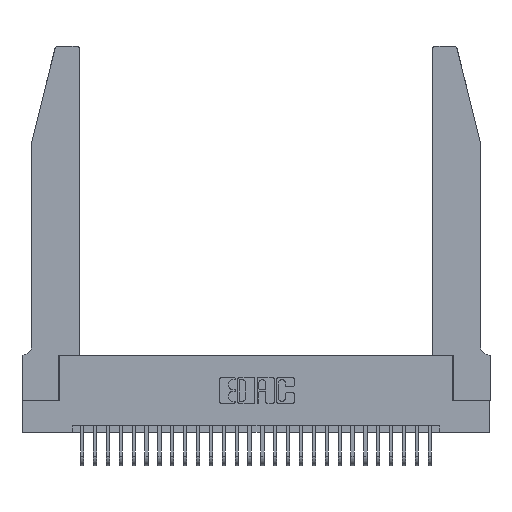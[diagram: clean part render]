
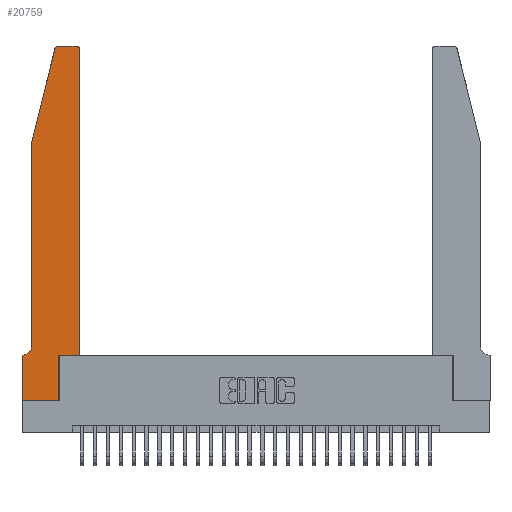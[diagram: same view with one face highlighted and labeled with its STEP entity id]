
A CAD part, top view. The second image highlights one B-rep face of the part: STEP entity #20759.
In plain terms, the highlighted planar face has unit normal (0, 0, 1).
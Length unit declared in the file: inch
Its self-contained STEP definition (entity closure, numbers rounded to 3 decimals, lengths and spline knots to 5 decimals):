
#238 = DIRECTION ( 'NONE',  ( 0., -1., 0. ) ) ;
#245 = CARTESIAN_POINT ( 'NONE',  ( 0.284, 2.72, 0.37 ) ) ;
#687 = VECTOR ( 'NONE', #22631, 39.37008 ) ;
#832 = CARTESIAN_POINT ( 'NONE',  ( 0.2865, 0.35, 0.37 ) ) ;
#835 = VERTEX_POINT ( 'NONE', #6418 ) ;
#898 = AXIS2_PLACEMENT_3D ( 'NONE', #245, #15365, #2438 ) ;
#1307 = VECTOR ( 'NONE', #238, 39.37008 ) ;
#1359 = LINE ( 'NONE', #5441, #687 ) ;
#1474 = EDGE_CURVE ( 'NONE', #16273, #2423, #24915, .T. ) ;
#1587 = ORIENTED_EDGE ( 'NONE', *, *, #12725, .T. ) ;
#1673 = EDGE_CURVE ( 'NONE', #17619, #4056, #3754, .T. ) ;
#2088 = VECTOR ( 'NONE', #20787, 39.37008 ) ;
#2423 = VERTEX_POINT ( 'NONE', #12526 ) ;
#2438 = DIRECTION ( 'NONE',  ( 1., 0., 0. ) ) ;
#2525 = ORIENTED_EDGE ( 'NONE', *, *, #5178, .T. ) ;
#2668 = DIRECTION ( 'NONE',  ( 0., 1., 0. ) ) ;
#2673 = DIRECTION ( 'NONE',  ( 1., 0., 0. ) ) ;
#2699 = VERTEX_POINT ( 'NONE', #11519 ) ;
#2999 = EDGE_LOOP ( 'NONE', ( #14582, #3633, #5471, #1587, #21951, #20219, #9209, #8102, #14599, #9055, #26476, #2525 ) ) ;
#3405 = VECTOR ( 'NONE', #24109, 39.37008 ) ;
#3633 = ORIENTED_EDGE ( 'NONE', *, *, #8452, .T. ) ;
#3653 = CIRCLE ( 'NONE', #20707, 0.03 ) ;
#3754 = LINE ( 'NONE', #13445, #5108 ) ;
#3864 = CIRCLE ( 'NONE', #7303, 0.07 ) ;
#3934 = EDGE_CURVE ( 'NONE', #6554, #13724, #21554, .T. ) ;
#4013 = VERTEX_POINT ( 'NONE', #22145 ) ;
#4056 = VERTEX_POINT ( 'NONE', #9401 ) ;
#4520 = CARTESIAN_POINT ( 'NONE',  ( 0.4205, 2.72, 0.37 ) ) ;
#4682 = VERTEX_POINT ( 'NONE', #832 ) ;
#5108 = VECTOR ( 'NONE', #2668, 39.37008 ) ;
#5178 = EDGE_CURVE ( 'NONE', #4056, #835, #3653, .T. ) ;
#5441 = CARTESIAN_POINT ( 'NONE',  ( 0.2865, 0.35, 0.37 ) ) ;
#5471 = ORIENTED_EDGE ( 'NONE', *, *, #3934, .T. ) ;
#5832 = CIRCLE ( 'NONE', #898, 0.03 ) ;
#6057 = CARTESIAN_POINT ( 'NONE',  ( 0., 0.35, 0.37 ) ) ;
#6418 = CARTESIAN_POINT ( 'NONE',  ( 0.4205, 2.75, 0.37 ) ) ;
#6554 = VERTEX_POINT ( 'NONE', #12341 ) ;
#6691 = DIRECTION ( 'NONE',  ( 1., 0., 0. ) ) ;
#6834 = DIRECTION ( 'NONE',  ( -1., 0., 0. ) ) ;
#6859 = CARTESIAN_POINT ( 'NONE',  ( 0.0755, 2., 0.37 ) ) ;
#7303 = AXIS2_PLACEMENT_3D ( 'NONE', #7445, #22435, #9608 ) ;
#7445 = CARTESIAN_POINT ( 'NONE',  ( 0.0055, 0.42, 0.37 ) ) ;
#7897 = EDGE_CURVE ( 'NONE', #835, #26061, #21327, .T. ) ;
#8102 = ORIENTED_EDGE ( 'NONE', *, *, #14953, .T. ) ;
#8213 = DIRECTION ( 'NONE',  ( 1., 0., 0. ) ) ;
#8452 = EDGE_CURVE ( 'NONE', #26061, #6554, #5832, .T. ) ;
#8543 = LINE ( 'NONE', #18635, #2088 ) ;
#8762 = PLANE ( 'NONE',  #12261 ) ;
#9055 = ORIENTED_EDGE ( 'NONE', *, *, #27440, .T. ) ;
#9209 = ORIENTED_EDGE ( 'NONE', *, *, #1474, .T. ) ;
#9401 = CARTESIAN_POINT ( 'NONE',  ( 0.4505, 2.72, 0.37 ) ) ;
#9608 = DIRECTION ( 'NONE',  ( -1., 0., 0. ) ) ;
#10051 = VECTOR ( 'NONE', #8213, 39.37008 ) ;
#10734 = CARTESIAN_POINT ( 'NONE',  ( 0., 0., 0.37 ) ) ;
#11048 = CARTESIAN_POINT ( 'NONE',  ( 0.0755, 2., 0.37 ) ) ;
#11202 = DIRECTION ( 'NONE',  ( -0.239, -0.971, 0. ) ) ;
#11519 = CARTESIAN_POINT ( 'NONE',  ( 0.0755, 0.42, 0.37 ) ) ;
#11924 = EDGE_CURVE ( 'NONE', #4013, #4682, #1359, .T. ) ;
#12261 = AXIS2_PLACEMENT_3D ( 'NONE', #24119, #15622, #2673 ) ;
#12341 = CARTESIAN_POINT ( 'NONE',  ( 0.25487, 2.72718, 0.37 ) ) ;
#12359 = CARTESIAN_POINT ( 'NONE',  ( 0.0755, 2., 0.37 ) ) ;
#12526 = CARTESIAN_POINT ( 'NONE',  ( 0., 0., 0.37 ) ) ;
#12725 = EDGE_CURVE ( 'NONE', #13724, #2699, #19181, .T. ) ;
#13445 = CARTESIAN_POINT ( 'NONE',  ( 0.4505, 0.35, 0.37 ) ) ;
#13724 = VERTEX_POINT ( 'NONE', #12359 ) ;
#13791 = VERTEX_POINT ( 'NONE', #25452 ) ;
#14582 = ORIENTED_EDGE ( 'NONE', *, *, #7897, .T. ) ;
#14599 = ORIENTED_EDGE ( 'NONE', *, *, #11924, .T. ) ;
#14722 = CARTESIAN_POINT ( 'NONE',  ( 0.284, 2.75, 0.37 ) ) ;
#14953 = EDGE_CURVE ( 'NONE', #2423, #4013, #21459, .T. ) ;
#15365 = DIRECTION ( 'NONE',  ( 0., 0., 1. ) ) ;
#15622 = DIRECTION ( 'NONE',  ( 0., 0., 1. ) ) ;
#16273 = VERTEX_POINT ( 'NONE', #6057 ) ;
#17551 = CARTESIAN_POINT ( 'NONE',  ( 0.2605, 2.75, 0.37 ) ) ;
#17619 = VERTEX_POINT ( 'NONE', #23547 ) ;
#18635 = CARTESIAN_POINT ( 'NONE',  ( 0.0755, 0.35, 0.37 ) ) ;
#19181 = LINE ( 'NONE', #11048, #1307 ) ;
#19563 = DIRECTION ( 'NONE',  ( 0., 0., 1. ) ) ;
#20219 = ORIENTED_EDGE ( 'NONE', *, *, #26601, .T. ) ;
#20573 = LINE ( 'NONE', #21950, #3405 ) ;
#20707 = AXIS2_PLACEMENT_3D ( 'NONE', #4520, #19563, #6691 ) ;
#20759 = ADVANCED_FACE ( 'NONE', ( #26899 ), #8762, .T. ) ;
#20787 = DIRECTION ( 'NONE',  ( -1., 0., 0. ) ) ;
#21327 = LINE ( 'NONE', #17551, #25635 ) ;
#21459 = LINE ( 'NONE', #27451, #10051 ) ;
#21554 = LINE ( 'NONE', #6859, #25876 ) ;
#21950 = CARTESIAN_POINT ( 'NONE',  ( 0.4505, 0.35, 0.37 ) ) ;
#21951 = ORIENTED_EDGE ( 'NONE', *, *, #24777, .T. ) ;
#22145 = CARTESIAN_POINT ( 'NONE',  ( 0.2865, 0., 0.37 ) ) ;
#22435 = DIRECTION ( 'NONE',  ( 0., 0., -1. ) ) ;
#22631 = DIRECTION ( 'NONE',  ( 0., 1., 0. ) ) ;
#23547 = CARTESIAN_POINT ( 'NONE',  ( 0.4505, 0.35, 0.37 ) ) ;
#24109 = DIRECTION ( 'NONE',  ( 1., 0., 0. ) ) ;
#24119 = CARTESIAN_POINT ( 'NONE',  ( 0., 0.35, 0.37 ) ) ;
#24777 = EDGE_CURVE ( 'NONE', #2699, #13791, #3864, .T. ) ;
#24915 = LINE ( 'NONE', #10734, #25565 ) ;
#25452 = CARTESIAN_POINT ( 'NONE',  ( 0.0055, 0.35, 0.37 ) ) ;
#25565 = VECTOR ( 'NONE', #25676, 39.37008 ) ;
#25635 = VECTOR ( 'NONE', #6834, 39.37008 ) ;
#25676 = DIRECTION ( 'NONE',  ( 0., -1., 0. ) ) ;
#25876 = VECTOR ( 'NONE', #11202, 39.37008 ) ;
#26061 = VERTEX_POINT ( 'NONE', #14722 ) ;
#26476 = ORIENTED_EDGE ( 'NONE', *, *, #1673, .T. ) ;
#26601 = EDGE_CURVE ( 'NONE', #13791, #16273, #8543, .T. ) ;
#26899 = FACE_OUTER_BOUND ( 'NONE', #2999, .T. ) ;
#27440 = EDGE_CURVE ( 'NONE', #4682, #17619, #20573, .T. ) ;
#27451 = CARTESIAN_POINT ( 'NONE',  ( 0., 0., 0.37 ) ) ;
